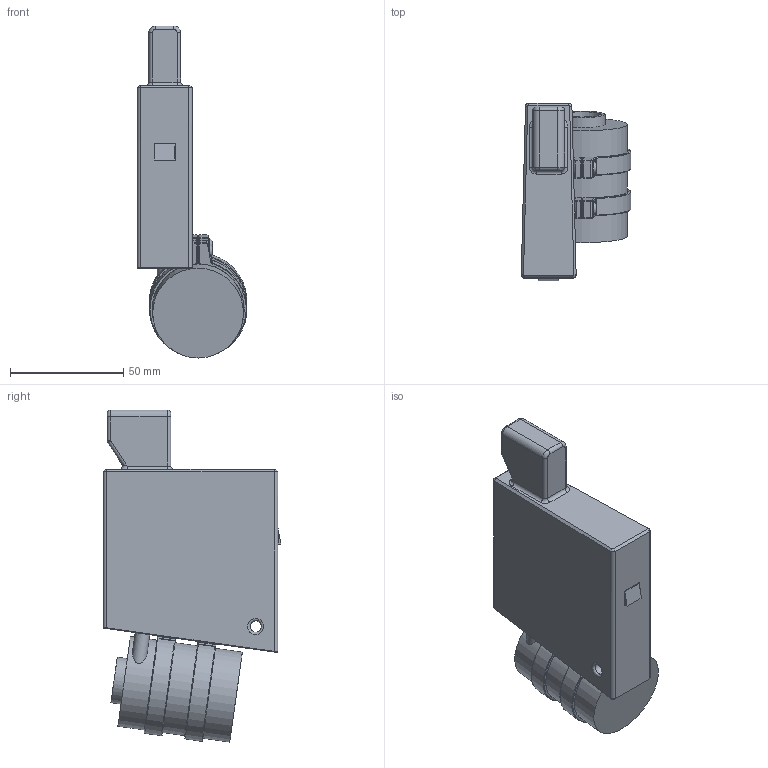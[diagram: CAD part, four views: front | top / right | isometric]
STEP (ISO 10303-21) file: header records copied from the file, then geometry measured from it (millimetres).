
FILE_DESCRIPTION(/* description */ (''),/* implementation_level */ '2;1');
FILE_NAME(/* name */ 'AW Active Cooling Magazine Block.step',/* time_stamp */ '2024-06-28T22:56:49+12:00',/* author */ (''),/* organization */ (''),/* preprocessor_version */ 'ST-DEVELOPER v20',/* originating_system */ 'Autodesk Translation Framework v13.14.0.145',/* authorisation */ '');
FILE_SCHEMA (('AUTOMOTIVE_DESIGN { 1 0 10303 214 3 1 1 }'));
Length unit declared in the file: millimetre
Products named in the file (3): AW Magazine Block; flextail_pump; M3x14 BHCS
Assembly tree (3 placements, depth 2):
  AW Magazine Block
    flextail_pump
    M3x14 BHCS  x2
Bounding box: 48.3 x 78.35 x 146.4 mm (x, y, z)
Volume: 203958 mm3; surface area: 38075.3 mm2
Topology: 6 solids, 6 shells, 287 faces, 617 edges, 358 vertices
Faces by surface type: cylinder 98, plane 81, bspline 56, torus 28, cone 20, sphere 4
Full cylindrical faces by diameter (mm): 2.8 x2, 3 x2, 3.4 x4, 5 x5, 5.7 x2, 6.5 x1, 6.8 x1, 16.8 x1, 20.2 x1, 40 x1
Entity records: 8876 total; most frequent: CARTESIAN_POINT 2963, DIRECTION 1278, ORIENTED_EDGE 1168, EDGE_CURVE 584, AXIS2_PLACEMENT_3D 518, VERTEX_POINT 340, EDGE_LOOP 292, FACE_OUTER_BOUND 267
